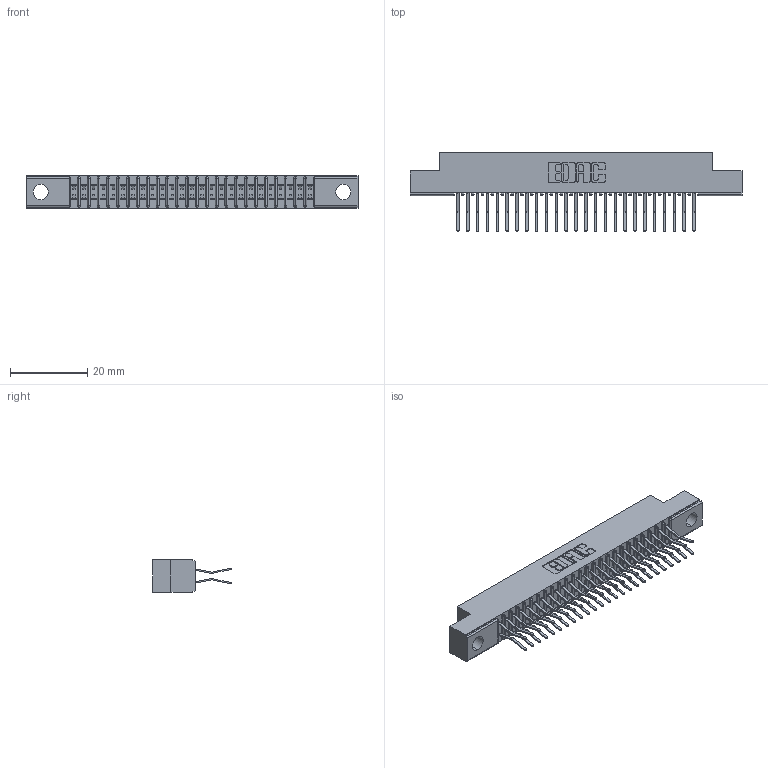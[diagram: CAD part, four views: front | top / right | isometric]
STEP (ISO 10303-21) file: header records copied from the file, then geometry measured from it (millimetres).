
FILE_DESCRIPTION (( 'STEP AP203' ), '1' );
FILE_NAME ('391-050-560-204.STEP', '2018-08-09T05:27:45', ( '' ), ( '' ), 'SwSTEP 2.0', 'SolidWorks 2016', '' );
FILE_SCHEMA (( 'CONFIG_CONTROL_DESIGN' ));
Length unit declared in the file: inch
Products named in the file (3): 391-050-560-204; 341 Part_.156 (3.96) Dia Mounting Holes; 341-292-001_341-292-160
Assembly tree (51 placements, depth 2):
  391-050-560-204
    341 Part_.156 (3.96) Dia Mounting Holes
    341-292-001_341-292-160  x50
Bounding box: 85.72 x 20.37 x 8.38 mm (x, y, z)
Volume: 4815.9 mm3; surface area: 10488.9 mm2
Topology: 51 solids, 51 shells, 3630 faces, 10527 edges, 6830 vertices
Faces by surface type: plane 2082, cylinder 1448, sphere 52, torus 48
Entity records: 33078 total; most frequent: CARTESIAN_POINT 5505, ORIENTED_EDGE 5466, DIRECTION 5351, EDGE_CURVE 2733, LINE 2191, VECTOR 2191, VERTEX_POINT 1734, AXIS2_PLACEMENT_3D 1580
